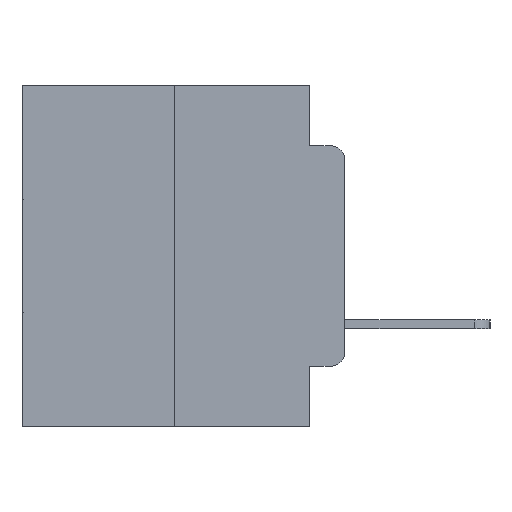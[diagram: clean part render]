
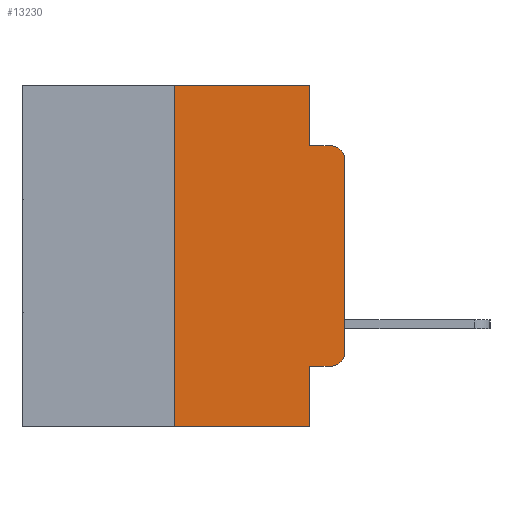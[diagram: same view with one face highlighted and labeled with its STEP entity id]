
A CAD part, left-side view. The second image highlights one B-rep face of the part: STEP entity #13230.
In plain terms, the highlighted planar face has unit normal (-1, 0, 0).
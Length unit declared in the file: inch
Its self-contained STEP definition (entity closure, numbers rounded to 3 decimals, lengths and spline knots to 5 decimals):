
#282 = EDGE_CURVE ( 'NONE', #19717, #11120, #23647, .T. ) ;
#508 = DIRECTION ( 'NONE',  ( 1., 0., 0. ) ) ;
#546 = VECTOR ( 'NONE', #25601, 39.37008 ) ;
#643 = VERTEX_POINT ( 'NONE', #1524 ) ;
#689 = CARTESIAN_POINT ( 'NONE',  ( 0., 0.25, 0. ) ) ;
#1524 = CARTESIAN_POINT ( 'NONE',  ( 0., 0., -0.3915 ) ) ;
#1757 = EDGE_CURVE ( 'NONE', #19717, #4213, #2002, .T. ) ;
#1778 = VERTEX_POINT ( 'NONE', #689 ) ;
#2002 = LINE ( 'NONE', #22046, #13685 ) ;
#2916 = CARTESIAN_POINT ( 'NONE',  ( 0., 0.051, -0.0885 ) ) ;
#2929 = EDGE_CURVE ( 'NONE', #1778, #5560, #12742, .T. ) ;
#3394 = AXIS2_PLACEMENT_3D ( 'NONE', #17700, #508, #15757 ) ;
#4213 = VERTEX_POINT ( 'NONE', #26326 ) ;
#4332 = VECTOR ( 'NONE', #24319, 39.37008 ) ;
#4477 = VECTOR ( 'NONE', #11127, 39.37008 ) ;
#4916 = ORIENTED_EDGE ( 'NONE', *, *, #13533, .T. ) ;
#5491 = CARTESIAN_POINT ( 'NONE',  ( 0., 0.02, -0.3915 ) ) ;
#5560 = VERTEX_POINT ( 'NONE', #17110 ) ;
#5715 = DIRECTION ( 'NONE',  ( 0., -1., 0. ) ) ;
#5722 = CARTESIAN_POINT ( 'NONE',  ( 0., 0.051, -0.4115 ) ) ;
#5807 = CARTESIAN_POINT ( 'NONE',  ( 0., 0.02, -0.0885 ) ) ;
#5819 = AXIS2_PLACEMENT_3D ( 'NONE', #5491, #21652, #9441 ) ;
#6310 = ORIENTED_EDGE ( 'NONE', *, *, #12098, .T. ) ;
#6330 = EDGE_CURVE ( 'NONE', #9092, #1778, #13496, .T. ) ;
#6555 = LINE ( 'NONE', #23572, #546 ) ;
#6881 = ORIENTED_EDGE ( 'NONE', *, *, #9272, .F. ) ;
#6908 = CARTESIAN_POINT ( 'NONE',  ( 0., 0.25, -0.5 ) ) ;
#6992 = ORIENTED_EDGE ( 'NONE', *, *, #7809, .F. ) ;
#7037 = VECTOR ( 'NONE', #23358, 39.37008 ) ;
#7168 = ORIENTED_EDGE ( 'NONE', *, *, #2929, .F. ) ;
#7339 = VECTOR ( 'NONE', #5715, 39.37008 ) ;
#7809 = EDGE_CURVE ( 'NONE', #5560, #15425, #6555, .T. ) ;
#7820 = VECTOR ( 'NONE', #14431, 39.37008 ) ;
#7874 = CARTESIAN_POINT ( 'NONE',  ( 0., 0.02, -0.1085 ) ) ;
#8080 = ORIENTED_EDGE ( 'NONE', *, *, #6330, .F. ) ;
#8791 = CARTESIAN_POINT ( 'NONE',  ( 0., 0., 0. ) ) ;
#8999 = CARTESIAN_POINT ( 'NONE',  ( 0., 0.473, -0.5 ) ) ;
#9092 = VERTEX_POINT ( 'NONE', #6908 ) ;
#9272 = EDGE_CURVE ( 'NONE', #15425, #16450, #26165, .T. ) ;
#9274 = CARTESIAN_POINT ( 'NONE',  ( 0., 0.051, -0.4115 ) ) ;
#9441 = DIRECTION ( 'NONE',  ( 0., 0., -1. ) ) ;
#10083 = DIRECTION ( 'NONE',  ( 0., 0., -1. ) ) ;
#10207 = CARTESIAN_POINT ( 'NONE',  ( 0., 0.25, 0. ) ) ;
#10724 = CARTESIAN_POINT ( 'NONE',  ( 0., 0., -0.1085 ) ) ;
#10943 = DIRECTION ( 'NONE',  ( 0., 0., 1. ) ) ;
#11120 = VERTEX_POINT ( 'NONE', #16149 ) ;
#11127 = DIRECTION ( 'NONE',  ( 0., -1., 0. ) ) ;
#11308 = CARTESIAN_POINT ( 'NONE',  ( 0., 0.473, 0. ) ) ;
#12098 = EDGE_CURVE ( 'NONE', #13045, #16450, #24837, .T. ) ;
#12742 = LINE ( 'NONE', #11308, #7037 ) ;
#13045 = VERTEX_POINT ( 'NONE', #10724 ) ;
#13230 = ADVANCED_FACE ( 'NONE', ( #18087 ), #23558, .F. ) ;
#13496 = LINE ( 'NONE', #10207, #7820 ) ;
#13533 = EDGE_CURVE ( 'NONE', #643, #13045, #25351, .T. ) ;
#13685 = VECTOR ( 'NONE', #16000, 39.37008 ) ;
#14387 = CARTESIAN_POINT ( 'NONE',  ( 0., 0.051, -0.0885 ) ) ;
#14431 = DIRECTION ( 'NONE',  ( 0., 0., 1. ) ) ;
#14897 = VECTOR ( 'NONE', #10943, 39.37008 ) ;
#15296 = EDGE_CURVE ( 'NONE', #9092, #4213, #15933, .T. ) ;
#15425 = VERTEX_POINT ( 'NONE', #2916 ) ;
#15757 = DIRECTION ( 'NONE',  ( 0., 0., -1. ) ) ;
#15933 = LINE ( 'NONE', #8999, #4477 ) ;
#16000 = DIRECTION ( 'NONE',  ( 0., 0., -1. ) ) ;
#16149 = CARTESIAN_POINT ( 'NONE',  ( 0., 0.02, -0.4115 ) ) ;
#16450 = VERTEX_POINT ( 'NONE', #5807 ) ;
#17110 = CARTESIAN_POINT ( 'NONE',  ( 0., 0.051, 0. ) ) ;
#17700 = CARTESIAN_POINT ( 'NONE',  ( 0., 0.473, 0. ) ) ;
#18087 = FACE_OUTER_BOUND ( 'NONE', #22505, .T. ) ;
#18611 = CIRCLE ( 'NONE', #5819, 0.02 ) ;
#19537 = ORIENTED_EDGE ( 'NONE', *, *, #1757, .F. ) ;
#19717 = VERTEX_POINT ( 'NONE', #9274 ) ;
#21145 = AXIS2_PLACEMENT_3D ( 'NONE', #7874, #22202, #10083 ) ;
#21252 = ORIENTED_EDGE ( 'NONE', *, *, #25956, .T. ) ;
#21652 = DIRECTION ( 'NONE',  ( -1., 0., 0. ) ) ;
#22046 = CARTESIAN_POINT ( 'NONE',  ( 0., 0.051, 0. ) ) ;
#22115 = ORIENTED_EDGE ( 'NONE', *, *, #282, .T. ) ;
#22202 = DIRECTION ( 'NONE',  ( -1., 0., 0. ) ) ;
#22505 = EDGE_LOOP ( 'NONE', ( #4916, #6310, #6881, #6992, #7168, #8080, #24112, #19537, #22115, #21252 ) ) ;
#23358 = DIRECTION ( 'NONE',  ( 0., -1., 0. ) ) ;
#23558 = PLANE ( 'NONE',  #3394 ) ;
#23572 = CARTESIAN_POINT ( 'NONE',  ( 0., 0.051, 0. ) ) ;
#23647 = LINE ( 'NONE', #5722, #7339 ) ;
#24112 = ORIENTED_EDGE ( 'NONE', *, *, #15296, .T. ) ;
#24319 = DIRECTION ( 'NONE',  ( 0., -1., 0. ) ) ;
#24837 = CIRCLE ( 'NONE', #21145, 0.02 ) ;
#25351 = LINE ( 'NONE', #8791, #14897 ) ;
#25601 = DIRECTION ( 'NONE',  ( 0., 0., -1. ) ) ;
#25956 = EDGE_CURVE ( 'NONE', #11120, #643, #18611, .T. ) ;
#26165 = LINE ( 'NONE', #14387, #4332 ) ;
#26326 = CARTESIAN_POINT ( 'NONE',  ( 0., 0.051, -0.5 ) ) ;
